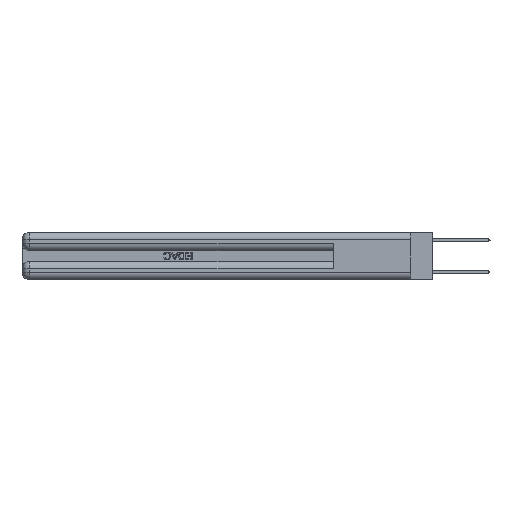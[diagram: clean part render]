
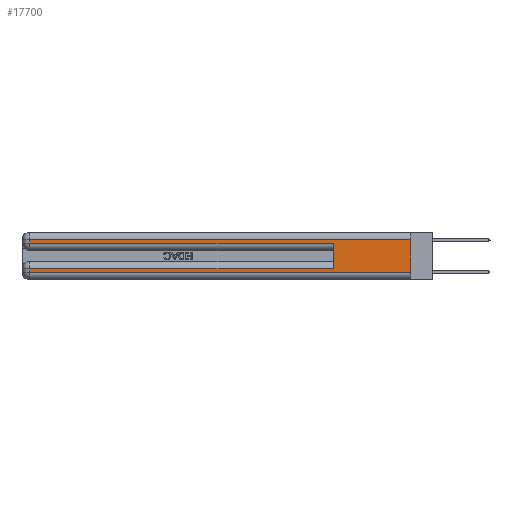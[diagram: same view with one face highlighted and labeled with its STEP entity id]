
A CAD part, left-side view. The second image highlights one B-rep face of the part: STEP entity #17700.
In plain terms, the highlighted planar face has unit normal (-1, 0, 0).
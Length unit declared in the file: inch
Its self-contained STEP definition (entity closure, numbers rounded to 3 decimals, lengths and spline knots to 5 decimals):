
#2080 = CARTESIAN_POINT ( 'NONE',  ( 0., 0., 0.31 ) ) ;
#2867 = LINE ( 'NONE', #15800, #23497 ) ;
#3106 = VERTEX_POINT ( 'NONE', #27913 ) ;
#3332 = VECTOR ( 'NONE', #6891, 39.37008 ) ;
#3347 = CARTESIAN_POINT ( 'NONE',  ( 0., 0., 0.085 ) ) ;
#3557 = VERTEX_POINT ( 'NONE', #6375 ) ;
#3948 = VERTEX_POINT ( 'NONE', #22523 ) ;
#4312 = CARTESIAN_POINT ( 'NONE',  ( 0., 0., 0.37 ) ) ;
#4434 = CARTESIAN_POINT ( 'NONE',  ( 0., 2.94, 0.31 ) ) ;
#4696 = DIRECTION ( 'NONE',  ( 0., 0., -1. ) ) ;
#4703 = DIRECTION ( 'NONE',  ( 0., 1., 0. ) ) ;
#4725 = ORIENTED_EDGE ( 'NONE', *, *, #22893, .T. ) ;
#5009 = LINE ( 'NONE', #17895, #23196 ) ;
#5055 = DIRECTION ( 'NONE',  ( 0., 0., -1. ) ) ;
#5063 = EDGE_CURVE ( 'NONE', #3106, #3557, #26031, .T. ) ;
#5953 = DIRECTION ( 'NONE',  ( 0., 1., 0. ) ) ;
#6179 = CARTESIAN_POINT ( 'NONE',  ( 0., 2.94, 0.285 ) ) ;
#6375 = CARTESIAN_POINT ( 'NONE',  ( 0., 0.6, 0.285 ) ) ;
#6402 = CARTESIAN_POINT ( 'NONE',  ( 0., 0., 0.285 ) ) ;
#6422 = VERTEX_POINT ( 'NONE', #25046 ) ;
#6457 = AXIS2_PLACEMENT_3D ( 'NONE', #12270, #30238, #14876 ) ;
#6464 = ORIENTED_EDGE ( 'NONE', *, *, #33148, .T. ) ;
#6610 = EDGE_LOOP ( 'NONE', ( #10680, #28444, #14931, #6464, #25108, #4725, #12648, #10627 ) ) ;
#6891 = DIRECTION ( 'NONE',  ( 0., 0., -1. ) ) ;
#7097 = VERTEX_POINT ( 'NONE', #7298 ) ;
#7298 = CARTESIAN_POINT ( 'NONE',  ( 0., 2.94, 0.085 ) ) ;
#9584 = LINE ( 'NONE', #22753, #29315 ) ;
#10452 = LINE ( 'NONE', #2080, #23413 ) ;
#10627 = ORIENTED_EDGE ( 'NONE', *, *, #26342, .T. ) ;
#10680 = ORIENTED_EDGE ( 'NONE', *, *, #24478, .F. ) ;
#11873 = EDGE_CURVE ( 'NONE', #7097, #6422, #9584, .T. ) ;
#12150 = PLANE ( 'NONE',  #6457 ) ;
#12270 = CARTESIAN_POINT ( 'NONE',  ( 0., 0., 0.37 ) ) ;
#12315 = VERTEX_POINT ( 'NONE', #4434 ) ;
#12648 = ORIENTED_EDGE ( 'NONE', *, *, #11873, .T. ) ;
#14059 = DIRECTION ( 'NONE',  ( 0., 0., 1. ) ) ;
#14876 = DIRECTION ( 'NONE',  ( 0., 0., -1. ) ) ;
#14931 = ORIENTED_EDGE ( 'NONE', *, *, #29736, .T. ) ;
#15800 = CARTESIAN_POINT ( 'NONE',  ( 0., 0., 0.06 ) ) ;
#15992 = LINE ( 'NONE', #3347, #28829 ) ;
#17499 = VERTEX_POINT ( 'NONE', #6179 ) ;
#17653 = LINE ( 'NONE', #6402, #24523 ) ;
#17700 = ADVANCED_FACE ( 'NONE', ( #23293 ), #12150, .F. ) ;
#17895 = CARTESIAN_POINT ( 'NONE',  ( 0., 2.94, 0.37 ) ) ;
#22523 = CARTESIAN_POINT ( 'NONE',  ( 0., 0., 0.06 ) ) ;
#22753 = CARTESIAN_POINT ( 'NONE',  ( 0., 2.94, 0.37 ) ) ;
#22893 = EDGE_CURVE ( 'NONE', #3106, #7097, #15992, .T. ) ;
#23196 = VECTOR ( 'NONE', #5055, 39.37008 ) ;
#23293 = FACE_OUTER_BOUND ( 'NONE', #6610, .T. ) ;
#23413 = VECTOR ( 'NONE', #4703, 39.37008 ) ;
#23497 = VECTOR ( 'NONE', #31144, 39.37008 ) ;
#23950 = LINE ( 'NONE', #4312, #3332 ) ;
#24467 = DIRECTION ( 'NONE',  ( 0., -1., 0. ) ) ;
#24478 = EDGE_CURVE ( 'NONE', #25841, #3948, #23950, .T. ) ;
#24523 = VECTOR ( 'NONE', #24467, 39.37008 ) ;
#25046 = CARTESIAN_POINT ( 'NONE',  ( 0., 2.94, 0.06 ) ) ;
#25108 = ORIENTED_EDGE ( 'NONE', *, *, #5063, .F. ) ;
#25841 = VERTEX_POINT ( 'NONE', #31614 ) ;
#26031 = LINE ( 'NONE', #32000, #32795 ) ;
#26342 = EDGE_CURVE ( 'NONE', #6422, #3948, #2867, .T. ) ;
#27913 = CARTESIAN_POINT ( 'NONE',  ( 0., 0.6, 0.085 ) ) ;
#28444 = ORIENTED_EDGE ( 'NONE', *, *, #32012, .T. ) ;
#28829 = VECTOR ( 'NONE', #5953, 39.37008 ) ;
#29315 = VECTOR ( 'NONE', #4696, 39.37008 ) ;
#29736 = EDGE_CURVE ( 'NONE', #12315, #17499, #5009, .T. ) ;
#30238 = DIRECTION ( 'NONE',  ( 1., 0., 0. ) ) ;
#31144 = DIRECTION ( 'NONE',  ( 0., -1., 0. ) ) ;
#31614 = CARTESIAN_POINT ( 'NONE',  ( 0., 0., 0.31 ) ) ;
#32000 = CARTESIAN_POINT ( 'NONE',  ( 0., 0.6, 0.145 ) ) ;
#32012 = EDGE_CURVE ( 'NONE', #25841, #12315, #10452, .T. ) ;
#32795 = VECTOR ( 'NONE', #14059, 39.37008 ) ;
#33148 = EDGE_CURVE ( 'NONE', #17499, #3557, #17653, .T. ) ;
